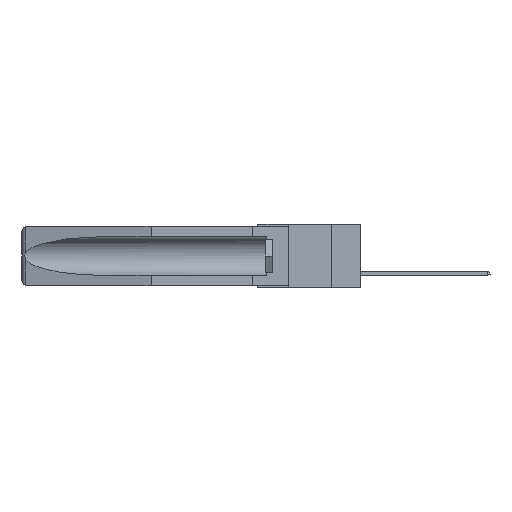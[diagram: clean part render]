
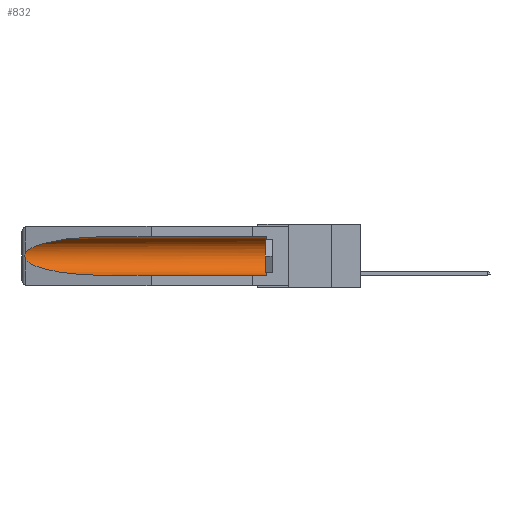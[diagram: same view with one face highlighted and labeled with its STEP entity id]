
A CAD part, left-side view. The second image highlights one B-rep face of the part: STEP entity #832.
In plain terms, the highlighted cylindrical face has radius 2.857 mm (diameter 5.715 mm), a partial arc.
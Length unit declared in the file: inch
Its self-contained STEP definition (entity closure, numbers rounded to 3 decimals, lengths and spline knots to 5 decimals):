
#821 = B_SPLINE_CURVE_WITH_KNOTS ( 'NONE', 3,
 ( #22396, #7262, #22304, #24569, #26873, #24471, #13894, #7080, #7370, #13704 ),
 .UNSPECIFIED., .F., .F.,
 ( 4, 2, 2, 2, 4 ),
 ( 0., 0.00029, 0.00058, 0.00087, 0.00117 ),
 .UNSPECIFIED. ) ;
#832 = ADVANCED_FACE ( 'NONE', ( #24571 ), #17865, .F. ) ;
#839 = CARTESIAN_POINT ( 'NONE',  ( 0.155, 0.126, -0.059 ) ) ;
#1035 = EDGE_CURVE ( 'NONE', #26545, #27928, #821, .T. ) ;
#1085 = ORIENTED_EDGE ( 'NONE', *, *, #16367, .F. ) ;
#1670 = CARTESIAN_POINT ( 'NONE',  ( 0.155, 1.07973, -0.059 ) ) ;
#1969 = CARTESIAN_POINT ( 'NONE',  ( 0.155, -0.30754, -0.059 ) ) ;
#2481 = ORIENTED_EDGE ( 'NONE', *, *, #21652, .T. ) ;
#2874 = CARTESIAN_POINT ( 'NONE',  ( 0.26537, 1.52718, -0.19328 ) ) ;
#3218 = CARTESIAN_POINT ( 'NONE',  ( 0.25451, 1.48313, -0.09465 ) ) ;
#3409 = VERTEX_POINT ( 'NONE', #10596 ) ;
#3525 = CARTESIAN_POINT ( 'NONE',  ( 0.25451, 1.48313, -0.24835 ) ) ;
#5087 = VERTEX_POINT ( 'NONE', #839 ) ;
#7080 = CARTESIAN_POINT ( 'NONE',  ( 0.26655, 1.53094, -0.18657 ) ) ;
#7262 = CARTESIAN_POINT ( 'NONE',  ( 0.26597, 1.52961, -0.15275 ) ) ;
#7370 = CARTESIAN_POINT ( 'NONE',  ( 0.26597, 1.5296, -0.19026 ) ) ;
#7519 = CARTESIAN_POINT ( 'NONE',  ( 0.21114, 1.30732, -0.059 ) ) ;
#7715 = CARTESIAN_POINT ( 'NONE',  ( 0.26537, 1.52718, -0.14972 ) ) ;
#8096 = LINE ( 'NONE', #23811, #16876 ) ;
#9932 = CARTESIAN_POINT ( 'NONE',  ( 0.155, 1.07973, -0.284 ) ) ;
#10596 = CARTESIAN_POINT ( 'NONE',  ( 0.155, 1.07973, -0.284 ) ) ;
#11680 = EDGE_CURVE ( 'NONE', #17690, #26545, #15579, .T. ) ;
#12139 =( BOUNDED_CURVE ( )  B_SPLINE_CURVE ( 3, ( #25230, #3525, #14451, #9932 ),
 .UNSPECIFIED., .F., .F. ) 
 B_SPLINE_CURVE_WITH_KNOTS ( ( 4, 4 ),
 ( 0.1948, 1.5708 ),
 .UNSPECIFIED. ) 
 CURVE ( )  GEOMETRIC_REPRESENTATION_ITEM ( )  RATIONAL_B_SPLINE_CURVE ( ( 1., 0.848, 0.848, 1. ) ) 
 REPRESENTATION_ITEM ( '' )  );
#12602 = DIRECTION ( 'NONE',  ( 0., 1., 0. ) ) ;
#13638 = CARTESIAN_POINT ( 'NONE',  ( 0.26537, 1.52718, -0.14972 ) ) ;
#13704 = CARTESIAN_POINT ( 'NONE',  ( 0.26537, 1.52718, -0.19328 ) ) ;
#13894 = CARTESIAN_POINT ( 'NONE',  ( 0.2673, 1.53269, -0.17917 ) ) ;
#14229 = CARTESIAN_POINT ( 'NONE',  ( 0.155, 1.07973, -0.059 ) ) ;
#14451 = CARTESIAN_POINT ( 'NONE',  ( 0.21114, 1.30732, -0.284 ) ) ;
#14496 = EDGE_CURVE ( 'NONE', #20509, #5087, #15993, .T. ) ;
#14584 = DIRECTION ( 'NONE',  ( 0., 0., 1. ) ) ;
#14796 = ORIENTED_EDGE ( 'NONE', *, *, #14496, .T. ) ;
#15037 = CARTESIAN_POINT ( 'NONE',  ( 0.155, -0.30754, -0.1715 ) ) ;
#15140 = ORIENTED_EDGE ( 'NONE', *, *, #11680, .T. ) ;
#15579 =( BOUNDED_CURVE ( )  B_SPLINE_CURVE ( 3, ( #14229, #7519, #3218, #7715 ),
 .UNSPECIFIED., .F., .F. ) 
 B_SPLINE_CURVE_WITH_KNOTS ( ( 4, 4 ),
 ( 4.71239, 6.08839 ),
 .UNSPECIFIED. ) 
 CURVE ( )  GEOMETRIC_REPRESENTATION_ITEM ( )  RATIONAL_B_SPLINE_CURVE ( ( 1., 0.848, 0.848, 1. ) ) 
 REPRESENTATION_ITEM ( '' )  );
#15993 = CIRCLE ( 'NONE', #26589, 0.1125 ) ;
#16367 = EDGE_CURVE ( 'NONE', #20509, #3409, #8096, .T. ) ;
#16876 = VECTOR ( 'NONE', #21760, 39.37008 ) ;
#17117 = DIRECTION ( 'NONE',  ( 0., 1., 0. ) ) ;
#17690 = VERTEX_POINT ( 'NONE', #1670 ) ;
#17865 = CYLINDRICAL_SURFACE ( 'NONE', #27462, 0.1125 ) ;
#20474 = VECTOR ( 'NONE', #12602, 39.37008 ) ;
#20509 = VERTEX_POINT ( 'NONE', #21881 ) ;
#21183 = EDGE_LOOP ( 'NONE', ( #15140, #21671, #26231, #1085, #14796, #2481 ) ) ;
#21380 = DIRECTION ( 'NONE',  ( 0., -1., 0. ) ) ;
#21652 = EDGE_CURVE ( 'NONE', #5087, #17690, #24513, .T. ) ;
#21659 = DIRECTION ( 'NONE',  ( 0., 0., 1. ) ) ;
#21671 = ORIENTED_EDGE ( 'NONE', *, *, #1035, .T. ) ;
#21760 = DIRECTION ( 'NONE',  ( 0., 1., 0. ) ) ;
#21881 = CARTESIAN_POINT ( 'NONE',  ( 0.155, 0.126, -0.284 ) ) ;
#22304 = CARTESIAN_POINT ( 'NONE',  ( 0.26654, 1.53092, -0.15636 ) ) ;
#22396 = CARTESIAN_POINT ( 'NONE',  ( 0.26537, 1.52718, -0.14972 ) ) ;
#22417 = EDGE_CURVE ( 'NONE', #27928, #3409, #12139, .T. ) ;
#23811 = CARTESIAN_POINT ( 'NONE',  ( 0.155, -0.30754, -0.284 ) ) ;
#24471 = CARTESIAN_POINT ( 'NONE',  ( 0.2675, 1.53308, -0.17534 ) ) ;
#24513 = LINE ( 'NONE', #1969, #20474 ) ;
#24569 = CARTESIAN_POINT ( 'NONE',  ( 0.2673, 1.5327, -0.16383 ) ) ;
#24571 = FACE_OUTER_BOUND ( 'NONE', #21183, .T. ) ;
#25230 = CARTESIAN_POINT ( 'NONE',  ( 0.26537, 1.52718, -0.19328 ) ) ;
#26231 = ORIENTED_EDGE ( 'NONE', *, *, #22417, .T. ) ;
#26545 = VERTEX_POINT ( 'NONE', #13638 ) ;
#26589 = AXIS2_PLACEMENT_3D ( 'NONE', #27741, #21380, #14584 ) ;
#26873 = CARTESIAN_POINT ( 'NONE',  ( 0.2675, 1.53308, -0.16763 ) ) ;
#27462 = AXIS2_PLACEMENT_3D ( 'NONE', #15037, #17117, #21659 ) ;
#27741 = CARTESIAN_POINT ( 'NONE',  ( 0.155, 0.126, -0.1715 ) ) ;
#27928 = VERTEX_POINT ( 'NONE', #2874 ) ;
